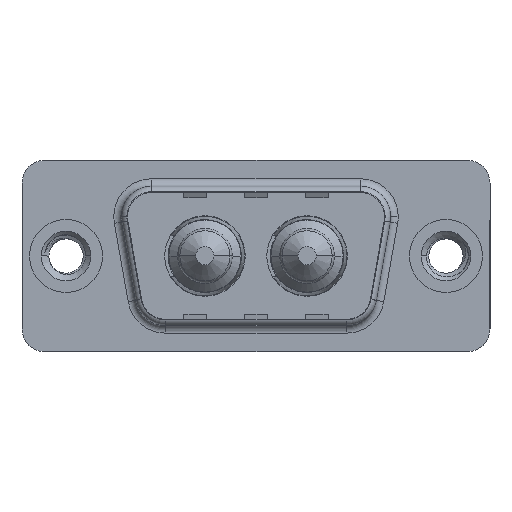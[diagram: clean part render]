
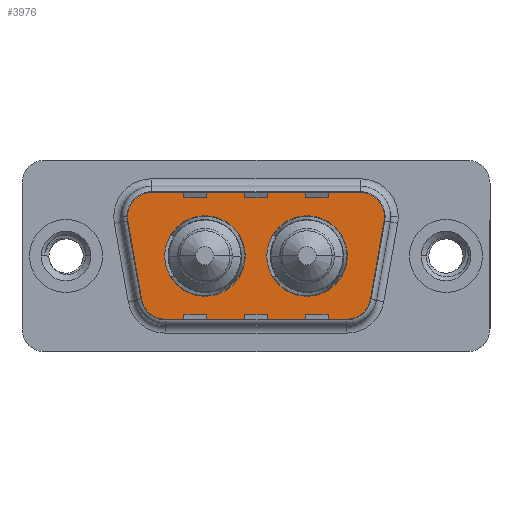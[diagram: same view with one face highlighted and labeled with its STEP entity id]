
A CAD part, top view. The second image highlights one B-rep face of the part: STEP entity #3976.
In plain terms, the highlighted planar face has unit normal (0, 0, 1).
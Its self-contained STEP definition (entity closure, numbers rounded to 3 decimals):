
#134 = CIRCLE ( 'NONE', #8486, 2. ) ;
#181 = VERTEX_POINT ( 'NONE', #5379 ) ;
#331 = CIRCLE ( 'NONE', #2464, 2.65 ) ;
#365 = VERTEX_POINT ( 'NONE', #7673 ) ;
#496 = EDGE_CURVE ( 'NONE', #11475, #4406, #331, .T. ) ;
#544 = CARTESIAN_POINT ( 'NONE',  ( 20.511, -3.247, 0. ) ) ;
#579 = ORIENTED_EDGE ( 'NONE', *, *, #12637, .F. ) ;
#594 = ORIENTED_EDGE ( 'NONE', *, *, #4319, .T. ) ;
#769 = ORIENTED_EDGE ( 'NONE', *, *, #12001, .T. ) ;
#1036 = CARTESIAN_POINT ( 'NONE',  ( 19.564, 2.9, 0. ) ) ;
#1151 = DIRECTION ( 'NONE',  ( 1., 0., 0. ) ) ;
#1283 = ORIENTED_EDGE ( 'NONE', *, *, #8155, .F. ) ;
#1438 = DIRECTION ( 'NONE',  ( 0., 0., 1. ) ) ;
#1453 = EDGE_CURVE ( 'NONE', #5839, #6139, #12128, .T. ) ;
#1582 = CARTESIAN_POINT ( 'NONE',  ( 6.459, -2.9, 0. ) ) ;
#1706 = FACE_BOUND ( 'NONE', #12475, .T. ) ;
#1777 = ORIENTED_EDGE ( 'NONE', *, *, #13724, .T. ) ;
#1822 = EDGE_CURVE ( 'NONE', #4574, #13886, #7502, .T. ) ;
#1903 = CARTESIAN_POINT ( 'NONE',  ( 19.564, 4.9, 0. ) ) ;
#2079 = DIRECTION ( 'NONE',  ( 0., 0., 1. ) ) ;
#2215 = CARTESIAN_POINT ( 'NONE',  ( 5.436, 2.9, 0. ) ) ;
#2464 = AXIS2_PLACEMENT_3D ( 'NONE', #11432, #1438, #1151 ) ;
#2533 = CARTESIAN_POINT ( 'NONE',  ( 15.86, 0., 0. ) ) ;
#2624 = CARTESIAN_POINT ( 'NONE',  ( 18.541, -2.9, 0. ) ) ;
#2664 = ORIENTED_EDGE ( 'NONE', *, *, #5733, .T. ) ;
#2667 = CARTESIAN_POINT ( 'NONE',  ( 21.564, 2.9, 0. ) ) ;
#2684 = DIRECTION ( 'NONE',  ( -1., 0., 0. ) ) ;
#2807 = DIRECTION ( 'NONE',  ( 0., 0., 1. ) ) ;
#3638 = DIRECTION ( 'NONE',  ( 1., 0., 0. ) ) ;
#3727 = DIRECTION ( 'NONE',  ( 1., 0., 0. ) ) ;
#3838 = CARTESIAN_POINT ( 'NONE',  ( 15.86, 0., 0. ) ) ;
#3912 = CIRCLE ( 'NONE', #14292, 2.65 ) ;
#3940 = DIRECTION ( 'NONE',  ( 0., 0., 1. ) ) ;
#3976 = ADVANCED_FACE ( 'NONE', ( #7618, #1706, #13269 ), #11326, .T. ) ;
#4319 = EDGE_CURVE ( 'NONE', #6139, #4574, #4480, .T. ) ;
#4403 = DIRECTION ( 'NONE',  ( 1., 0., 0. ) ) ;
#4406 = VERTEX_POINT ( 'NONE', #7958 ) ;
#4480 = LINE ( 'NONE', #11327, #13085 ) ;
#4534 = AXIS2_PLACEMENT_3D ( 'NONE', #9000, #9105, #10043 ) ;
#4574 = VERTEX_POINT ( 'NONE', #10447 ) ;
#4792 = AXIS2_PLACEMENT_3D ( 'NONE', #2215, #2807, #13350 ) ;
#4920 = AXIS2_PLACEMENT_3D ( 'NONE', #2624, #10461, #3727 ) ;
#4965 = DIRECTION ( 'NONE',  ( 1., 0., 0. ) ) ;
#5177 = CARTESIAN_POINT ( 'NONE',  ( 21.534, 2.553, 0. ) ) ;
#5190 = AXIS2_PLACEMENT_3D ( 'NONE', #8788, #2079, #9920 ) ;
#5332 = CIRCLE ( 'NONE', #5190, 2. ) ;
#5379 = CARTESIAN_POINT ( 'NONE',  ( 6.459, -4.9, 0. ) ) ;
#5557 = DIRECTION ( 'NONE',  ( -1., 0., 0. ) ) ;
#5733 = EDGE_CURVE ( 'NONE', #181, #9287, #6054, .T. ) ;
#5808 = DIRECTION ( 'NONE',  ( 0.174, -0.985, 0. ) ) ;
#5839 = VERTEX_POINT ( 'NONE', #2667 ) ;
#5881 = VECTOR ( 'NONE', #5808, 1000. ) ;
#5996 = DIRECTION ( 'NONE',  ( -1., 0., 0. ) ) ;
#6054 = LINE ( 'NONE', #12340, #8673 ) ;
#6139 = VERTEX_POINT ( 'NONE', #1903 ) ;
#6259 = CARTESIAN_POINT ( 'NONE',  ( 18.51, 0., 0. ) ) ;
#6626 = EDGE_LOOP ( 'NONE', ( #1283, #11447 ) ) ;
#6903 = LINE ( 'NONE', #5177, #9897 ) ;
#7077 = CIRCLE ( 'NONE', #4920, 2. ) ;
#7306 = CARTESIAN_POINT ( 'NONE',  ( 11.79, 0., 0. ) ) ;
#7502 = CIRCLE ( 'NONE', #4792, 2. ) ;
#7618 = FACE_BOUND ( 'NONE', #6626, .T. ) ;
#7673 = CARTESIAN_POINT ( 'NONE',  ( 13.21, 0., 0. ) ) ;
#7810 = CARTESIAN_POINT ( 'NONE',  ( 21.534, 2.553, 0. ) ) ;
#7829 = CIRCLE ( 'NONE', #12399, 2.65 ) ;
#7958 = CARTESIAN_POINT ( 'NONE',  ( 6.49, 0., 0. ) ) ;
#8128 = CIRCLE ( 'NONE', #11097, 2.65 ) ;
#8155 = EDGE_CURVE ( 'NONE', #9326, #365, #8128, .T. ) ;
#8486 = AXIS2_PLACEMENT_3D ( 'NONE', #1582, #9386, #2684 ) ;
#8673 = VECTOR ( 'NONE', #4403, 1000. ) ;
#8751 = ORIENTED_EDGE ( 'NONE', *, *, #11691, .T. ) ;
#8788 = CARTESIAN_POINT ( 'NONE',  ( 19.564, 2.9, 0. ) ) ;
#9000 = CARTESIAN_POINT ( 'NONE',  ( 18.541, -2.9, 0. ) ) ;
#9105 = DIRECTION ( 'NONE',  ( 0., 0., 1. ) ) ;
#9196 = VERTEX_POINT ( 'NONE', #544 ) ;
#9287 = VERTEX_POINT ( 'NONE', #14022 ) ;
#9326 = VERTEX_POINT ( 'NONE', #6259 ) ;
#9386 = DIRECTION ( 'NONE',  ( 0., 0., 1. ) ) ;
#9647 = VERTEX_POINT ( 'NONE', #12392 ) ;
#9768 = DIRECTION ( 'NONE',  ( 0., 0., 1. ) ) ;
#9866 = AXIS2_PLACEMENT_3D ( 'NONE', #1036, #9768, #5996 ) ;
#9897 = VECTOR ( 'NONE', #13061, 1000. ) ;
#9920 = DIRECTION ( 'NONE',  ( -1., 0., 0. ) ) ;
#10043 = DIRECTION ( 'NONE',  ( 1., 0., 0. ) ) ;
#10394 = DIRECTION ( 'NONE',  ( 0., 0., 1. ) ) ;
#10447 = CARTESIAN_POINT ( 'NONE',  ( 5.436, 4.9, 0. ) ) ;
#10461 = DIRECTION ( 'NONE',  ( 0., 0., 1. ) ) ;
#10631 = EDGE_CURVE ( 'NONE', #365, #9326, #7829, .T. ) ;
#10713 = CARTESIAN_POINT ( 'NONE',  ( 9.14, 0., 0. ) ) ;
#11065 = VERTEX_POINT ( 'NONE', #7810 ) ;
#11089 = ORIENTED_EDGE ( 'NONE', *, *, #1453, .T. ) ;
#11097 = AXIS2_PLACEMENT_3D ( 'NONE', #2533, #10394, #3638 ) ;
#11326 = PLANE ( 'NONE',  #4534 ) ;
#11327 = CARTESIAN_POINT ( 'NONE',  ( 5.436, 4.9, 0. ) ) ;
#11432 = CARTESIAN_POINT ( 'NONE',  ( 9.14, 0., 0. ) ) ;
#11445 = CARTESIAN_POINT ( 'NONE',  ( 3.466, 2.553, 0. ) ) ;
#11447 = ORIENTED_EDGE ( 'NONE', *, *, #10631, .F. ) ;
#11475 = VERTEX_POINT ( 'NONE', #7306 ) ;
#11661 = ORIENTED_EDGE ( 'NONE', *, *, #1822, .T. ) ;
#11691 = EDGE_CURVE ( 'NONE', #11065, #5839, #5332, .T. ) ;
#11719 = DIRECTION ( 'NONE',  ( 0., 0., 1. ) ) ;
#11848 = DIRECTION ( 'NONE',  ( 1., 0., 0. ) ) ;
#11875 = LINE ( 'NONE', #13640, #5881 ) ;
#12001 = EDGE_CURVE ( 'NONE', #13886, #9647, #11875, .T. ) ;
#12128 = CIRCLE ( 'NONE', #9866, 2. ) ;
#12319 = ORIENTED_EDGE ( 'NONE', *, *, #13347, .T. ) ;
#12340 = CARTESIAN_POINT ( 'NONE',  ( 6.459, -4.9, 0. ) ) ;
#12392 = CARTESIAN_POINT ( 'NONE',  ( 4.489, -3.247, 0. ) ) ;
#12399 = AXIS2_PLACEMENT_3D ( 'NONE', #3838, #11719, #4965 ) ;
#12475 = EDGE_LOOP ( 'NONE', ( #14198, #579 ) ) ;
#12637 = EDGE_CURVE ( 'NONE', #4406, #11475, #3912, .T. ) ;
#12690 = EDGE_LOOP ( 'NONE', ( #1777, #12319, #8751, #11089, #594, #11661, #769, #13703, #2664 ) ) ;
#13061 = DIRECTION ( 'NONE',  ( 0.174, 0.985, 0. ) ) ;
#13062 = EDGE_CURVE ( 'NONE', #9647, #181, #134, .T. ) ;
#13085 = VECTOR ( 'NONE', #5557, 1000. ) ;
#13269 = FACE_OUTER_BOUND ( 'NONE', #12690, .T. ) ;
#13347 = EDGE_CURVE ( 'NONE', #9196, #11065, #6903, .T. ) ;
#13350 = DIRECTION ( 'NONE',  ( 1., 0., 0. ) ) ;
#13640 = CARTESIAN_POINT ( 'NONE',  ( 3.466, 2.553, 0. ) ) ;
#13703 = ORIENTED_EDGE ( 'NONE', *, *, #13062, .T. ) ;
#13724 = EDGE_CURVE ( 'NONE', #9287, #9196, #7077, .T. ) ;
#13886 = VERTEX_POINT ( 'NONE', #11445 ) ;
#14022 = CARTESIAN_POINT ( 'NONE',  ( 18.541, -4.9, 0. ) ) ;
#14198 = ORIENTED_EDGE ( 'NONE', *, *, #496, .F. ) ;
#14292 = AXIS2_PLACEMENT_3D ( 'NONE', #10713, #3940, #11848 ) ;
